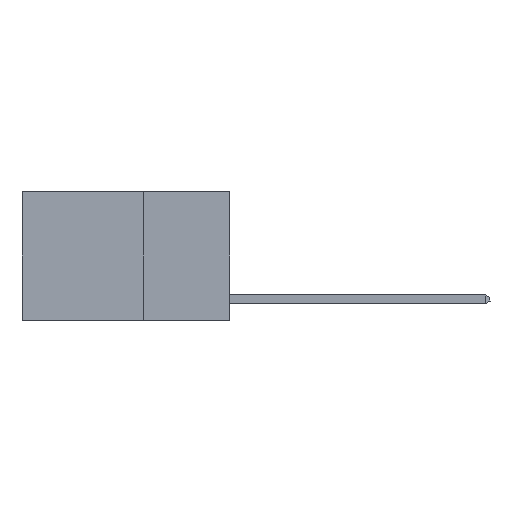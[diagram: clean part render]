
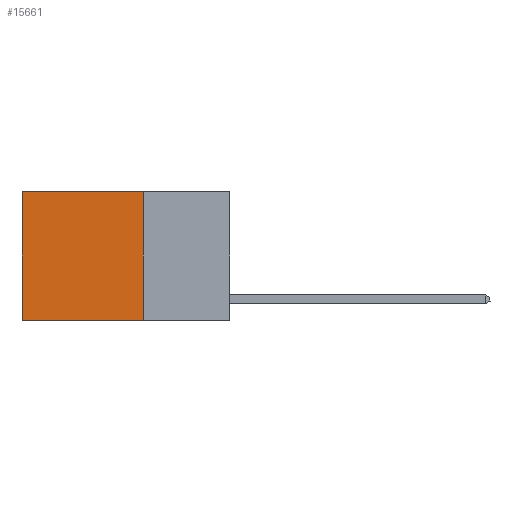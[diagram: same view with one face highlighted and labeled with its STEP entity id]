
A CAD part, left-side view. The second image highlights one B-rep face of the part: STEP entity #15661.
In plain terms, the highlighted planar face has unit normal (-1, 0, 0).
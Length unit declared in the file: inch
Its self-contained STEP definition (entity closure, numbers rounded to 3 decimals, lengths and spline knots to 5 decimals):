
#1136 = DIRECTION ( 'NONE',  ( 1., 0., 0. ) ) ;
#1923 = VECTOR ( 'NONE', #8860, 39.37008 ) ;
#2640 = VERTEX_POINT ( 'NONE', #15834 ) ;
#2728 = EDGE_CURVE ( 'NONE', #2640, #8607, #7383, .T. ) ;
#2822 = AXIS2_PLACEMENT_3D ( 'NONE', #17745, #1136, #10922 ) ;
#2997 = EDGE_CURVE ( 'NONE', #8607, #3582, #4809, .T. ) ;
#3012 = LINE ( 'NONE', #10447, #13166 ) ;
#3073 = ORIENTED_EDGE ( 'NONE', *, *, #5402, .F. ) ;
#3582 = VERTEX_POINT ( 'NONE', #9361 ) ;
#3610 = DIRECTION ( 'NONE',  ( 0., 1., 0. ) ) ;
#3748 = VECTOR ( 'NONE', #9092, 39.37008 ) ;
#3958 = DIRECTION ( 'NONE',  ( 0., 0., -1. ) ) ;
#4809 = LINE ( 'NONE', #14984, #6079 ) ;
#5402 = EDGE_CURVE ( 'NONE', #12304, #3582, #3012, .T. ) ;
#6079 = VECTOR ( 'NONE', #3958, 39.37008 ) ;
#6101 = ORIENTED_EDGE ( 'NONE', *, *, #2728, .T. ) ;
#7383 = LINE ( 'NONE', #15999, #3748 ) ;
#7510 = CARTESIAN_POINT ( 'NONE',  ( 0.2625, 0.25, 0. ) ) ;
#8607 = VERTEX_POINT ( 'NONE', #17846 ) ;
#8860 = DIRECTION ( 'NONE',  ( 0., 0., -1. ) ) ;
#9092 = DIRECTION ( 'NONE',  ( 0., 1., 0. ) ) ;
#9210 = CARTESIAN_POINT ( 'NONE',  ( 0.2625, 0.25, -0.37 ) ) ;
#9361 = CARTESIAN_POINT ( 'NONE',  ( 0.2625, 0.6, -0.37 ) ) ;
#10416 = FACE_OUTER_BOUND ( 'NONE', #11545, .T. ) ;
#10447 = CARTESIAN_POINT ( 'NONE',  ( 0.2625, 0.25, -0.37 ) ) ;
#10922 = DIRECTION ( 'NONE',  ( 0., 0., -1. ) ) ;
#11545 = EDGE_LOOP ( 'NONE', ( #12961, #3073, #16448, #6101 ) ) ;
#12304 = VERTEX_POINT ( 'NONE', #9210 ) ;
#12961 = ORIENTED_EDGE ( 'NONE', *, *, #2997, .T. ) ;
#13050 = LINE ( 'NONE', #7510, #1923 ) ;
#13166 = VECTOR ( 'NONE', #3610, 39.37008 ) ;
#14984 = CARTESIAN_POINT ( 'NONE',  ( 0.2625, 0.6, 0. ) ) ;
#15661 = ADVANCED_FACE ( 'NONE', ( #10416 ), #16405, .F. ) ;
#15834 = CARTESIAN_POINT ( 'NONE',  ( 0.2625, 0.25, 0. ) ) ;
#15999 = CARTESIAN_POINT ( 'NONE',  ( 0.2625, 0.25, 0. ) ) ;
#16405 = PLANE ( 'NONE',  #2822 ) ;
#16448 = ORIENTED_EDGE ( 'NONE', *, *, #16798, .F. ) ;
#16798 = EDGE_CURVE ( 'NONE', #2640, #12304, #13050, .T. ) ;
#17745 = CARTESIAN_POINT ( 'NONE',  ( 0.2625, 0.25, 0. ) ) ;
#17846 = CARTESIAN_POINT ( 'NONE',  ( 0.2625, 0.6, 0. ) ) ;
